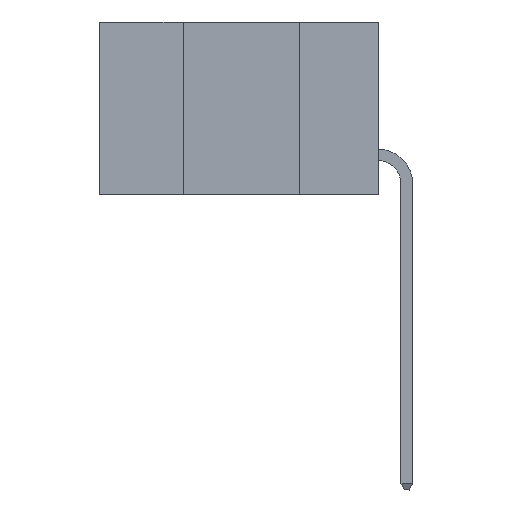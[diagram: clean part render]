
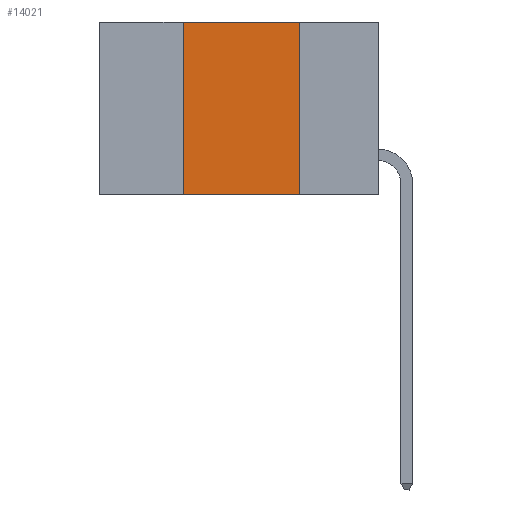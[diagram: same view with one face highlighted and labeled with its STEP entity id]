
A CAD part, left-side view. The second image highlights one B-rep face of the part: STEP entity #14021.
In plain terms, the highlighted planar face has unit normal (-1, 0, 0).
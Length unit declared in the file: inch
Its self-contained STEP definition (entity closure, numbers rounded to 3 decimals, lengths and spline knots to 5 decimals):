
#771 = VECTOR ( 'NONE', #4173, 39.37008 ) ;
#2237 = ORIENTED_EDGE ( 'NONE', *, *, #4159, .T. ) ;
#3577 = DIRECTION ( 'NONE',  ( 0., 0., -1. ) ) ;
#4113 = CARTESIAN_POINT ( 'NONE',  ( 0., 0.6, -0.37 ) ) ;
#4159 = EDGE_CURVE ( 'NONE', #12090, #4962, #4782, .T. ) ;
#4173 = DIRECTION ( 'NONE',  ( 0., -1., 0. ) ) ;
#4744 = VECTOR ( 'NONE', #11079, 39.37008 ) ;
#4782 = LINE ( 'NONE', #4113, #771 ) ;
#4962 = VERTEX_POINT ( 'NONE', #5503 ) ;
#5156 = VERTEX_POINT ( 'NONE', #9230 ) ;
#5503 = CARTESIAN_POINT ( 'NONE',  ( 0., 0.17, -0.37 ) ) ;
#5974 = CARTESIAN_POINT ( 'NONE',  ( 0., 0.6, 0. ) ) ;
#6308 = DIRECTION ( 'NONE',  ( 0., 0., 1. ) ) ;
#7365 = ORIENTED_EDGE ( 'NONE', *, *, #16395, .F. ) ;
#8055 = CARTESIAN_POINT ( 'NONE',  ( 0., 0.17, 0. ) ) ;
#9230 = CARTESIAN_POINT ( 'NONE',  ( 0., 0.17, 0. ) ) ;
#10267 = CARTESIAN_POINT ( 'NONE',  ( 0., 0.42, -0.37 ) ) ;
#11079 = DIRECTION ( 'NONE',  ( 0., 0., -1. ) ) ;
#11602 = ORIENTED_EDGE ( 'NONE', *, *, #15844, .F. ) ;
#12090 = VERTEX_POINT ( 'NONE', #10267 ) ;
#12495 = EDGE_LOOP ( 'NONE', ( #13617, #7365, #11602, #2237 ) ) ;
#12911 = FACE_OUTER_BOUND ( 'NONE', #12495, .T. ) ;
#12967 = VERTEX_POINT ( 'NONE', #14181 ) ;
#13043 = LINE ( 'NONE', #5974, #14296 ) ;
#13048 = DIRECTION ( 'NONE',  ( 1., 0., 0. ) ) ;
#13216 = EDGE_CURVE ( 'NONE', #5156, #4962, #13990, .T. ) ;
#13617 = ORIENTED_EDGE ( 'NONE', *, *, #13216, .F. ) ;
#13873 = DIRECTION ( 'NONE',  ( 0., -1., 0. ) ) ;
#13990 = LINE ( 'NONE', #8055, #4744 ) ;
#14021 = ADVANCED_FACE ( 'NONE', ( #12911 ), #15591, .F. ) ;
#14181 = CARTESIAN_POINT ( 'NONE',  ( 0., 0.42, 0. ) ) ;
#14296 = VECTOR ( 'NONE', #13873, 39.37008 ) ;
#14489 = CARTESIAN_POINT ( 'NONE',  ( 0., 0.42, 0. ) ) ;
#14585 = AXIS2_PLACEMENT_3D ( 'NONE', #17027, #13048, #3577 ) ;
#14936 = VECTOR ( 'NONE', #6308, 39.37008 ) ;
#15591 = PLANE ( 'NONE',  #14585 ) ;
#15844 = EDGE_CURVE ( 'NONE', #12090, #12967, #16374, .T. ) ;
#16374 = LINE ( 'NONE', #14489, #14936 ) ;
#16395 = EDGE_CURVE ( 'NONE', #12967, #5156, #13043, .T. ) ;
#17027 = CARTESIAN_POINT ( 'NONE',  ( 0., 0.6, 0. ) ) ;
